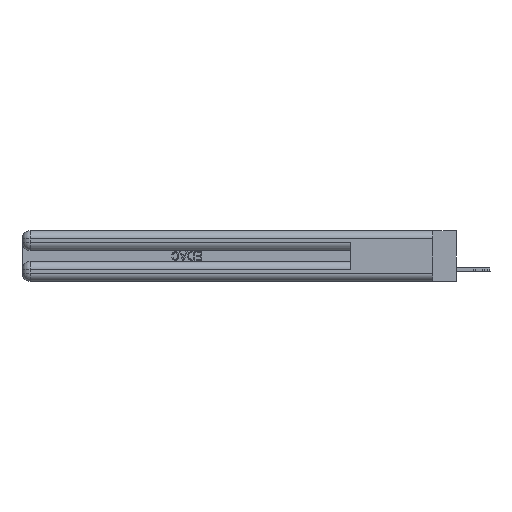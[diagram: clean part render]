
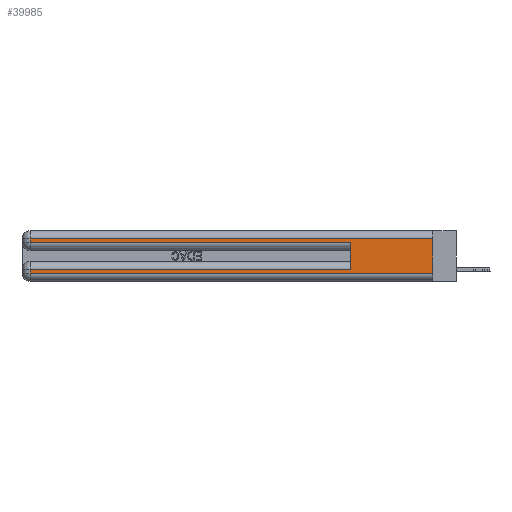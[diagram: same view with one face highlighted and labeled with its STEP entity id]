
A CAD part, left-side view. The second image highlights one B-rep face of the part: STEP entity #39985.
In plain terms, the highlighted planar face has unit normal (-1, 0, 0).
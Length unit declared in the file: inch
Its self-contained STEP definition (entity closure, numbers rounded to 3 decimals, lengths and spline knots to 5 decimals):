
#284 = VECTOR ( 'NONE', #23760, 39.37008 ) ;
#603 = CARTESIAN_POINT ( 'NONE',  ( 0., 2.94, 0.37 ) ) ;
#1612 = CARTESIAN_POINT ( 'NONE',  ( 0., 0.6, 0.085 ) ) ;
#1735 = VECTOR ( 'NONE', #28623, 39.37008 ) ;
#2459 = ORIENTED_EDGE ( 'NONE', *, *, #14217, .T. ) ;
#2683 = LINE ( 'NONE', #47917, #12619 ) ;
#2984 = CARTESIAN_POINT ( 'NONE',  ( 0., 0., 0.31 ) ) ;
#5698 = EDGE_LOOP ( 'NONE', ( #46752, #2459, #11574, #12525, #44587, #7435, #41494, #26829 ) ) ;
#6312 = VECTOR ( 'NONE', #20759, 39.37008 ) ;
#6779 = CARTESIAN_POINT ( 'NONE',  ( 0., 0., 0.37 ) ) ;
#7030 = VECTOR ( 'NONE', #28141, 39.37008 ) ;
#7435 = ORIENTED_EDGE ( 'NONE', *, *, #41793, .T. ) ;
#9551 = CARTESIAN_POINT ( 'NONE',  ( 0., 0.6, 0.145 ) ) ;
#9732 = VERTEX_POINT ( 'NONE', #41241 ) ;
#10076 = VECTOR ( 'NONE', #34260, 39.37008 ) ;
#10444 = DIRECTION ( 'NONE',  ( 0., 0., -1. ) ) ;
#10950 = LINE ( 'NONE', #9551, #284 ) ;
#11574 = ORIENTED_EDGE ( 'NONE', *, *, #30911, .T. ) ;
#11906 = CARTESIAN_POINT ( 'NONE',  ( 0., 0., 0.06 ) ) ;
#12525 = ORIENTED_EDGE ( 'NONE', *, *, #30683, .T. ) ;
#12619 = VECTOR ( 'NONE', #28153, 39.37008 ) ;
#14174 = DIRECTION ( 'NONE',  ( 0., 0., -1. ) ) ;
#14217 = EDGE_CURVE ( 'NONE', #24586, #26904, #40633, .T. ) ;
#19595 = FACE_OUTER_BOUND ( 'NONE', #5698, .T. ) ;
#19949 = EDGE_CURVE ( 'NONE', #45070, #30041, #33533, .T. ) ;
#20613 = LINE ( 'NONE', #43919, #7030 ) ;
#20759 = DIRECTION ( 'NONE',  ( 0., -1., 0. ) ) ;
#23623 = AXIS2_PLACEMENT_3D ( 'NONE', #6779, #30460, #10444 ) ;
#23760 = DIRECTION ( 'NONE',  ( 0., 0., 1. ) ) ;
#24278 = CARTESIAN_POINT ( 'NONE',  ( 0., 0., 0.37 ) ) ;
#24353 = LINE ( 'NONE', #24278, #10076 ) ;
#24586 = VERTEX_POINT ( 'NONE', #2984 ) ;
#24618 = CARTESIAN_POINT ( 'NONE',  ( 0., 2.94, 0.37 ) ) ;
#26829 = ORIENTED_EDGE ( 'NONE', *, *, #28901, .T. ) ;
#26904 = VERTEX_POINT ( 'NONE', #27035 ) ;
#27035 = CARTESIAN_POINT ( 'NONE',  ( 0., 2.94, 0.31 ) ) ;
#28141 = DIRECTION ( 'NONE',  ( 0., 1., 0. ) ) ;
#28153 = DIRECTION ( 'NONE',  ( 0., -1., 0. ) ) ;
#28415 = CARTESIAN_POINT ( 'NONE',  ( 0., 2.94, 0.285 ) ) ;
#28623 = DIRECTION ( 'NONE',  ( 0., 0., -1. ) ) ;
#28901 = EDGE_CURVE ( 'NONE', #30041, #46967, #2683, .T. ) ;
#29562 = VERTEX_POINT ( 'NONE', #1612 ) ;
#30041 = VERTEX_POINT ( 'NONE', #37563 ) ;
#30426 = EDGE_CURVE ( 'NONE', #24586, #46967, #24353, .T. ) ;
#30460 = DIRECTION ( 'NONE',  ( 1., 0., 0. ) ) ;
#30683 = EDGE_CURVE ( 'NONE', #42353, #9732, #43791, .T. ) ;
#30911 = EDGE_CURVE ( 'NONE', #26904, #42353, #47501, .T. ) ;
#31240 = VECTOR ( 'NONE', #32746, 39.37008 ) ;
#32746 = DIRECTION ( 'NONE',  ( 0., 1., 0. ) ) ;
#33533 = LINE ( 'NONE', #603, #1735 ) ;
#33700 = EDGE_CURVE ( 'NONE', #29562, #9732, #10950, .T. ) ;
#34260 = DIRECTION ( 'NONE',  ( 0., 0., -1. ) ) ;
#34326 = VECTOR ( 'NONE', #14174, 39.37008 ) ;
#36757 = CARTESIAN_POINT ( 'NONE',  ( 0., 0., 0.285 ) ) ;
#37563 = CARTESIAN_POINT ( 'NONE',  ( 0., 2.94, 0.06 ) ) ;
#39985 = ADVANCED_FACE ( 'NONE', ( #19595 ), #50374, .F. ) ;
#40633 = LINE ( 'NONE', #48667, #31240 ) ;
#41241 = CARTESIAN_POINT ( 'NONE',  ( 0., 0.6, 0.285 ) ) ;
#41494 = ORIENTED_EDGE ( 'NONE', *, *, #19949, .T. ) ;
#41793 = EDGE_CURVE ( 'NONE', #29562, #45070, #20613, .T. ) ;
#41803 = CARTESIAN_POINT ( 'NONE',  ( 0., 2.94, 0.085 ) ) ;
#42353 = VERTEX_POINT ( 'NONE', #28415 ) ;
#43791 = LINE ( 'NONE', #36757, #6312 ) ;
#43919 = CARTESIAN_POINT ( 'NONE',  ( 0., 0., 0.085 ) ) ;
#44587 = ORIENTED_EDGE ( 'NONE', *, *, #33700, .F. ) ;
#45070 = VERTEX_POINT ( 'NONE', #41803 ) ;
#46752 = ORIENTED_EDGE ( 'NONE', *, *, #30426, .F. ) ;
#46967 = VERTEX_POINT ( 'NONE', #11906 ) ;
#47501 = LINE ( 'NONE', #24618, #34326 ) ;
#47917 = CARTESIAN_POINT ( 'NONE',  ( 0., 0., 0.06 ) ) ;
#48667 = CARTESIAN_POINT ( 'NONE',  ( 0., 0., 0.31 ) ) ;
#50374 = PLANE ( 'NONE',  #23623 ) ;
